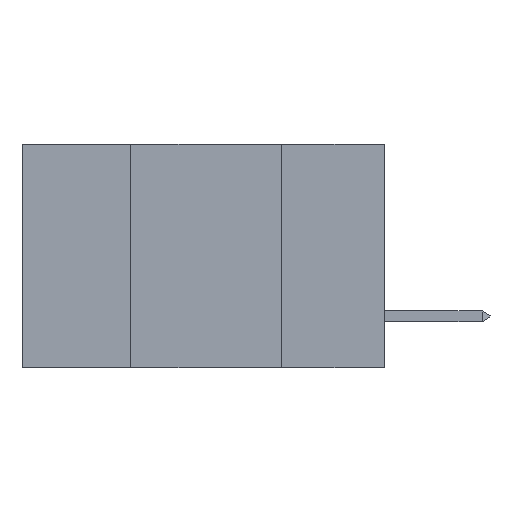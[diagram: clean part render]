
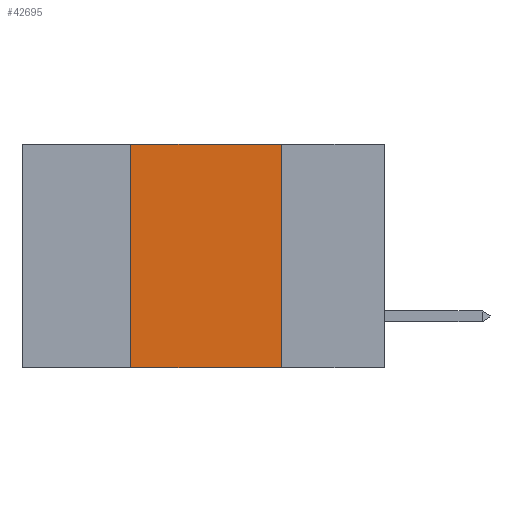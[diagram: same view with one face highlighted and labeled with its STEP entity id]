
A CAD part, left-side view. The second image highlights one B-rep face of the part: STEP entity #42695.
In plain terms, the highlighted planar face has unit normal (-1, 0, 0).
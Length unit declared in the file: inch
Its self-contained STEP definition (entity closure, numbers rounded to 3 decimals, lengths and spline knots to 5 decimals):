
#635 = EDGE_CURVE ( 'NONE', #9695, #21029, #30412, .T. ) ;
#1481 = ORIENTED_EDGE ( 'NONE', *, *, #17259, .T. ) ;
#2551 = LINE ( 'NONE', #36741, #33073 ) ;
#4943 = DIRECTION ( 'NONE',  ( 0., 0., -1. ) ) ;
#6544 = EDGE_LOOP ( 'NONE', ( #6702, #15133, #17871, #1481 ) ) ;
#6702 = ORIENTED_EDGE ( 'NONE', *, *, #42510, .F. ) ;
#9695 = VERTEX_POINT ( 'NONE', #20609 ) ;
#11447 = CARTESIAN_POINT ( 'NONE',  ( 0., 0.17, -0.37 ) ) ;
#13109 = LINE ( 'NONE', #39850, #21143 ) ;
#14697 = DIRECTION ( 'NONE',  ( 0., -1., 0. ) ) ;
#15133 = ORIENTED_EDGE ( 'NONE', *, *, #16415, .F. ) ;
#16415 = EDGE_CURVE ( 'NONE', #21029, #45304, #13109, .T. ) ;
#16807 = CARTESIAN_POINT ( 'NONE',  ( 0., 0.42, 0. ) ) ;
#17259 = EDGE_CURVE ( 'NONE', #9695, #24360, #2551, .T. ) ;
#17671 = DIRECTION ( 'NONE',  ( 0., 0., -1. ) ) ;
#17871 = ORIENTED_EDGE ( 'NONE', *, *, #635, .F. ) ;
#17919 = VECTOR ( 'NONE', #17671, 39.37008 ) ;
#20609 = CARTESIAN_POINT ( 'NONE',  ( 0., 0.42, -0.37 ) ) ;
#21029 = VERTEX_POINT ( 'NONE', #16807 ) ;
#21133 = AXIS2_PLACEMENT_3D ( 'NONE', #48630, #26066, #4943 ) ;
#21143 = VECTOR ( 'NONE', #39598, 39.37008 ) ;
#21372 = CARTESIAN_POINT ( 'NONE',  ( 0., 0.17, 0. ) ) ;
#23211 = CARTESIAN_POINT ( 'NONE',  ( 0., 0.42, 0. ) ) ;
#24360 = VERTEX_POINT ( 'NONE', #11447 ) ;
#26066 = DIRECTION ( 'NONE',  ( 1., 0., 0. ) ) ;
#29067 = LINE ( 'NONE', #21372, #17919 ) ;
#29946 = VECTOR ( 'NONE', #34372, 39.37008 ) ;
#30412 = LINE ( 'NONE', #23211, #29946 ) ;
#33073 = VECTOR ( 'NONE', #14697, 39.37008 ) ;
#33995 = PLANE ( 'NONE',  #21133 ) ;
#34372 = DIRECTION ( 'NONE',  ( 0., 0., 1. ) ) ;
#36741 = CARTESIAN_POINT ( 'NONE',  ( 0., 0.6, -0.37 ) ) ;
#39598 = DIRECTION ( 'NONE',  ( 0., -1., 0. ) ) ;
#39670 = CARTESIAN_POINT ( 'NONE',  ( 0., 0.17, 0. ) ) ;
#39850 = CARTESIAN_POINT ( 'NONE',  ( 0., 0.6, 0. ) ) ;
#42510 = EDGE_CURVE ( 'NONE', #45304, #24360, #29067, .T. ) ;
#42603 = FACE_OUTER_BOUND ( 'NONE', #6544, .T. ) ;
#42695 = ADVANCED_FACE ( 'NONE', ( #42603 ), #33995, .F. ) ;
#45304 = VERTEX_POINT ( 'NONE', #39670 ) ;
#48630 = CARTESIAN_POINT ( 'NONE',  ( 0., 0.6, 0. ) ) ;
